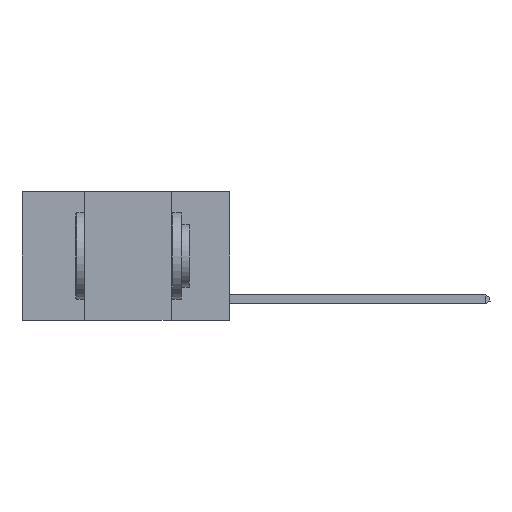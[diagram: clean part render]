
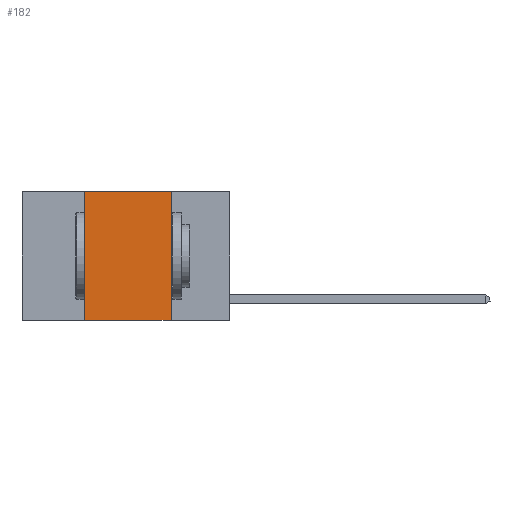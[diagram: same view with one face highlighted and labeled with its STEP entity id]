
A CAD part, left-side view. The second image highlights one B-rep face of the part: STEP entity #182.
In plain terms, the highlighted planar face has unit normal (-1, 0, 0).
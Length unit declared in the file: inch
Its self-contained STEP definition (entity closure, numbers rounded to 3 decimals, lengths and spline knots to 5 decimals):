
#76 = DIRECTION ( 'NONE',  ( 0., 0., -1. ) ) ;
#182 = ADVANCED_FACE ( 'NONE', ( #4118 ), #18637, .F. ) ;
#381 = EDGE_CURVE ( 'NONE', #15890, #5314, #12492, .T. ) ;
#930 = CARTESIAN_POINT ( 'NONE',  ( 0., 0.42, 0. ) ) ;
#1166 = EDGE_CURVE ( 'NONE', #16229, #8867, #14294, .T. ) ;
#1517 = DIRECTION ( 'NONE',  ( 0., -1., 0. ) ) ;
#1878 = ORIENTED_EDGE ( 'NONE', *, *, #1166, .F. ) ;
#2077 = VECTOR ( 'NONE', #1517, 39.37008 ) ;
#2471 = DIRECTION ( 'NONE',  ( 0., 0., 1. ) ) ;
#2756 = DIRECTION ( 'NONE',  ( 0., 0., -1. ) ) ;
#2928 = CARTESIAN_POINT ( 'NONE',  ( 0., 0.42, 0. ) ) ;
#3588 = ORIENTED_EDGE ( 'NONE', *, *, #13844, .F. ) ;
#4118 = FACE_OUTER_BOUND ( 'NONE', #17152, .T. ) ;
#5134 = ORIENTED_EDGE ( 'NONE', *, *, #15649, .F. ) ;
#5193 = CARTESIAN_POINT ( 'NONE',  ( 0., 0.6, 0. ) ) ;
#5314 = VERTEX_POINT ( 'NONE', #13876 ) ;
#6778 = AXIS2_PLACEMENT_3D ( 'NONE', #16980, #13535, #2756 ) ;
#7559 = CARTESIAN_POINT ( 'NONE',  ( 0., 0.17, 0. ) ) ;
#8867 = VERTEX_POINT ( 'NONE', #16620 ) ;
#9910 = CARTESIAN_POINT ( 'NONE',  ( 0., 0.42, -0.37 ) ) ;
#10826 = VECTOR ( 'NONE', #76, 39.37008 ) ;
#11049 = CARTESIAN_POINT ( 'NONE',  ( 0., 0.6, -0.37 ) ) ;
#12492 = LINE ( 'NONE', #11049, #2077 ) ;
#13535 = DIRECTION ( 'NONE',  ( 1., 0., 0. ) ) ;
#13844 = EDGE_CURVE ( 'NONE', #15890, #16229, #18165, .T. ) ;
#13876 = CARTESIAN_POINT ( 'NONE',  ( 0., 0.17, -0.37 ) ) ;
#14130 = VECTOR ( 'NONE', #2471, 39.37008 ) ;
#14294 = LINE ( 'NONE', #5193, #17473 ) ;
#14513 = DIRECTION ( 'NONE',  ( 0., -1., 0. ) ) ;
#15649 = EDGE_CURVE ( 'NONE', #8867, #5314, #20401, .T. ) ;
#15890 = VERTEX_POINT ( 'NONE', #9910 ) ;
#16115 = ORIENTED_EDGE ( 'NONE', *, *, #381, .T. ) ;
#16229 = VERTEX_POINT ( 'NONE', #2928 ) ;
#16620 = CARTESIAN_POINT ( 'NONE',  ( 0., 0.17, 0. ) ) ;
#16980 = CARTESIAN_POINT ( 'NONE',  ( 0., 0.6, 0. ) ) ;
#17152 = EDGE_LOOP ( 'NONE', ( #5134, #1878, #3588, #16115 ) ) ;
#17473 = VECTOR ( 'NONE', #14513, 39.37008 ) ;
#18165 = LINE ( 'NONE', #930, #14130 ) ;
#18637 = PLANE ( 'NONE',  #6778 ) ;
#20401 = LINE ( 'NONE', #7559, #10826 ) ;
